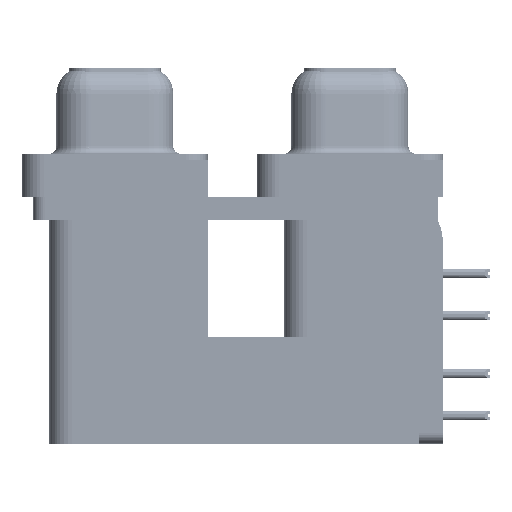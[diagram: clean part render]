
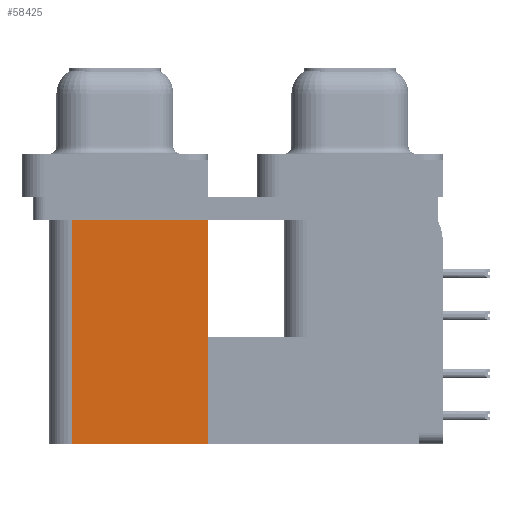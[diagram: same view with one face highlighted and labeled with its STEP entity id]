
A CAD part, left-side view. The second image highlights one B-rep face of the part: STEP entity #58425.
In plain terms, the highlighted planar face has unit normal (-1, 0, 0).
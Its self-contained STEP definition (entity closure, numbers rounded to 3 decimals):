
#975 = CARTESIAN_POINT ( 'NONE',  ( 3.79, 9.6, -19.2 ) ) ;
#5663 = AXIS2_PLACEMENT_3D ( 'NONE', #975, #28500, #23953 ) ;
#8149 = LINE ( 'NONE', #71060, #35499 ) ;
#8908 = CARTESIAN_POINT ( 'NONE',  ( 3.79, 9.6, -19.2 ) ) ;
#12634 = FACE_OUTER_BOUND ( 'NONE', #74251, .T. ) ;
#12688 = DIRECTION ( 'NONE',  ( 0., 1., 0. ) ) ;
#13649 = EDGE_CURVE ( 'NONE', #70448, #66565, #14109, .T. ) ;
#13808 = DIRECTION ( 'NONE',  ( 0., 0., 1. ) ) ;
#14109 = LINE ( 'NONE', #60078, #34337 ) ;
#15057 = EDGE_CURVE ( 'NONE', #25014, #70448, #68575, .T. ) ;
#18035 = CARTESIAN_POINT ( 'NONE',  ( 3.79, 9.6, -2.5 ) ) ;
#18043 = CARTESIAN_POINT ( 'NONE',  ( 3.79, 18.8, -19.2 ) ) ;
#18749 = EDGE_CURVE ( 'NONE', #25014, #64300, #8149, .T. ) ;
#19639 = LINE ( 'NONE', #47538, #34562 ) ;
#19854 = VECTOR ( 'NONE', #12688, 1000. ) ;
#23953 = DIRECTION ( 'NONE',  ( 0., 0., -1. ) ) ;
#25014 = VERTEX_POINT ( 'NONE', #8908 ) ;
#28024 = ORIENTED_EDGE ( 'NONE', *, *, #13649, .F. ) ;
#28500 = DIRECTION ( 'NONE',  ( 1., 0., 0. ) ) ;
#30737 = ORIENTED_EDGE ( 'NONE', *, *, #56429, .T. ) ;
#34337 = VECTOR ( 'NONE', #58972, 1000. ) ;
#34562 = VECTOR ( 'NONE', #58493, 1000. ) ;
#35499 = VECTOR ( 'NONE', #13808, 1000. ) ;
#45598 = CARTESIAN_POINT ( 'NONE',  ( 3.79, 9.6, -19.2 ) ) ;
#46210 = ORIENTED_EDGE ( 'NONE', *, *, #15057, .F. ) ;
#47538 = CARTESIAN_POINT ( 'NONE',  ( 3.79, 9.6, -2.5 ) ) ;
#56429 = EDGE_CURVE ( 'NONE', #64300, #66565, #19639, .T. ) ;
#58425 = ADVANCED_FACE ( 'NONE', ( #12634 ), #69171, .F. ) ;
#58493 = DIRECTION ( 'NONE',  ( 0., 1., 0. ) ) ;
#58972 = DIRECTION ( 'NONE',  ( 0., 0., 1. ) ) ;
#60078 = CARTESIAN_POINT ( 'NONE',  ( 3.79, 18.8, -19.2 ) ) ;
#64300 = VERTEX_POINT ( 'NONE', #18035 ) ;
#66565 = VERTEX_POINT ( 'NONE', #73435 ) ;
#68548 = ORIENTED_EDGE ( 'NONE', *, *, #18749, .T. ) ;
#68575 = LINE ( 'NONE', #45598, #19854 ) ;
#69171 = PLANE ( 'NONE',  #5663 ) ;
#70448 = VERTEX_POINT ( 'NONE', #18043 ) ;
#71060 = CARTESIAN_POINT ( 'NONE',  ( 3.79, 9.6, -19.2 ) ) ;
#73435 = CARTESIAN_POINT ( 'NONE',  ( 3.79, 18.8, -2.5 ) ) ;
#74251 = EDGE_LOOP ( 'NONE', ( #30737, #28024, #46210, #68548 ) ) ;
